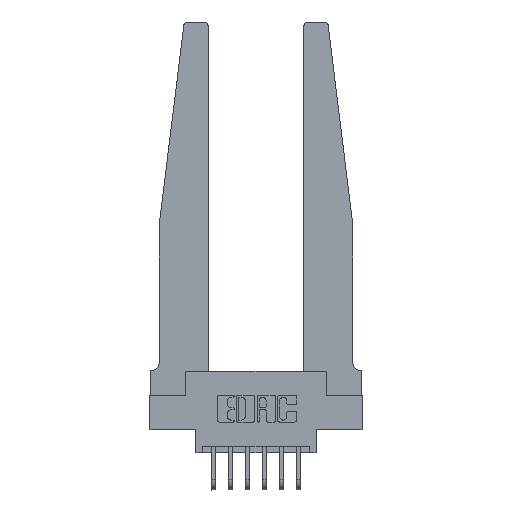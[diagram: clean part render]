
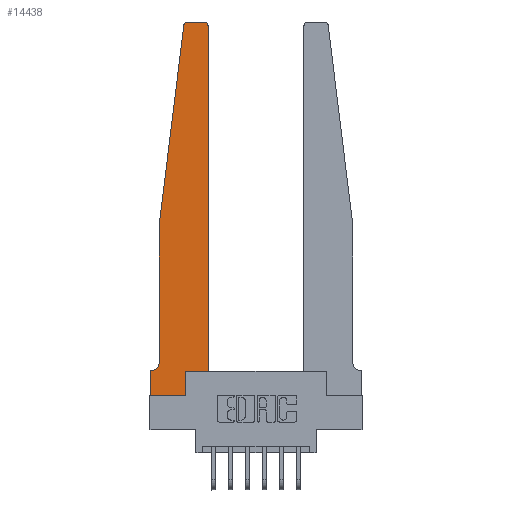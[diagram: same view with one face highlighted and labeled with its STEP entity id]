
A CAD part, top view. The second image highlights one B-rep face of the part: STEP entity #14438.
In plain terms, the highlighted planar face has unit normal (0, 0, 1).
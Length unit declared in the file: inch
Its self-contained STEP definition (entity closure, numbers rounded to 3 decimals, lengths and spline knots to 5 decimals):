
#33 = CARTESIAN_POINT ( 'NONE',  ( 0.2605, 0.18, 0.37 ) ) ;
#292 = CARTESIAN_POINT ( 'NONE',  ( 0.2605, 0.18, 0.37 ) ) ;
#530 = EDGE_CURVE ( 'NONE', #10565, #9992, #12898, .T. ) ;
#574 = ORIENTED_EDGE ( 'NONE', *, *, #530, .T. ) ;
#736 = CARTESIAN_POINT ( 'NONE',  ( 0.24675, 2.72367, 0.37 ) ) ;
#763 = VECTOR ( 'NONE', #12219, 39.37008 ) ;
#827 = VERTEX_POINT ( 'NONE', #8592 ) ;
#1291 = LINE ( 'NONE', #292, #8267 ) ;
#1582 = DIRECTION ( 'NONE',  ( 1., 0., 0. ) ) ;
#1612 = ORIENTED_EDGE ( 'NONE', *, *, #15298, .T. ) ;
#1615 = VERTEX_POINT ( 'NONE', #8436 ) ;
#1773 = EDGE_CURVE ( 'NONE', #827, #10565, #1291, .T. ) ;
#1791 = DIRECTION ( 'NONE',  ( 1., 0., 0. ) ) ;
#1896 = CIRCLE ( 'NONE', #10002, 0.05 ) ;
#2230 = LINE ( 'NONE', #6598, #2796 ) ;
#2315 = CARTESIAN_POINT ( 'NONE',  ( 0.27653, 2.75, 0.37 ) ) ;
#2355 = ORIENTED_EDGE ( 'NONE', *, *, #10225, .T. ) ;
#2376 = DIRECTION ( 'NONE',  ( 1., 0., 0. ) ) ;
#2778 = CARTESIAN_POINT ( 'NONE',  ( 0.425, 0.18, 0.37 ) ) ;
#2796 = VECTOR ( 'NONE', #7716, 39.37008 ) ;
#3054 = DIRECTION ( 'NONE',  ( -1., 0., 0. ) ) ;
#3140 = DIRECTION ( 'NONE',  ( 1., 0., 0. ) ) ;
#3184 = VERTEX_POINT ( 'NONE', #10871 ) ;
#3187 = DIRECTION ( 'NONE',  ( 0., -1., 0. ) ) ;
#3250 = CARTESIAN_POINT ( 'NONE',  ( 0., 0., 0.37 ) ) ;
#3554 = ORIENTED_EDGE ( 'NONE', *, *, #5472, .T. ) ;
#3602 = CARTESIAN_POINT ( 'NONE',  ( 0.27653, 2.72, 0.37 ) ) ;
#3672 = ORIENTED_EDGE ( 'NONE', *, *, #7025, .T. ) ;
#4065 = CARTESIAN_POINT ( 'NONE',  ( 0., 0., 0.37 ) ) ;
#4136 = FACE_OUTER_BOUND ( 'NONE', #4164, .T. ) ;
#4147 = CARTESIAN_POINT ( 'NONE',  ( 0.065, 1.25, 0.37 ) ) ;
#4158 = LINE ( 'NONE', #13344, #8698 ) ;
#4164 = EDGE_LOOP ( 'NONE', ( #13473, #2355, #3672, #8071, #6270, #7700, #9556, #3554, #5638, #574, #1612, #5847 ) ) ;
#4544 = AXIS2_PLACEMENT_3D ( 'NONE', #3602, #11991, #1582 ) ;
#4931 = VECTOR ( 'NONE', #11007, 39.37008 ) ;
#5241 = LINE ( 'NONE', #7638, #9429 ) ;
#5472 = EDGE_CURVE ( 'NONE', #8073, #827, #13823, .T. ) ;
#5638 = ORIENTED_EDGE ( 'NONE', *, *, #1773, .T. ) ;
#5847 = ORIENTED_EDGE ( 'NONE', *, *, #10850, .T. ) ;
#6134 = DIRECTION ( 'NONE',  ( 0., 1., 0. ) ) ;
#6270 = ORIENTED_EDGE ( 'NONE', *, *, #9929, .T. ) ;
#6478 = LINE ( 'NONE', #7479, #4931 ) ;
#6598 = CARTESIAN_POINT ( 'NONE',  ( 0.25, 2.75, 0.37 ) ) ;
#6753 = CARTESIAN_POINT ( 'NONE',  ( 0.395, 2.75, 0.37 ) ) ;
#6863 = PLANE ( 'NONE',  #7045 ) ;
#6876 = AXIS2_PLACEMENT_3D ( 'NONE', #14218, #14267, #2376 ) ;
#6998 = DIRECTION ( 'NONE',  ( 0., 0., -1. ) ) ;
#7025 = EDGE_CURVE ( 'NONE', #13683, #13902, #6478, .T. ) ;
#7045 = AXIS2_PLACEMENT_3D ( 'NONE', #9255, #7933, #3140 ) ;
#7364 = EDGE_CURVE ( 'NONE', #14016, #8073, #13776, .T. ) ;
#7479 = CARTESIAN_POINT ( 'NONE',  ( 0.065, 1.25, 0.37 ) ) ;
#7638 = CARTESIAN_POINT ( 'NONE',  ( 0.065, 1.25, 0.37 ) ) ;
#7700 = ORIENTED_EDGE ( 'NONE', *, *, #10220, .T. ) ;
#7716 = DIRECTION ( 'NONE',  ( -1., 0., 0. ) ) ;
#7933 = DIRECTION ( 'NONE',  ( 0., 0., 1. ) ) ;
#8071 = ORIENTED_EDGE ( 'NONE', *, *, #10265, .T. ) ;
#8073 = VERTEX_POINT ( 'NONE', #15427 ) ;
#8267 = VECTOR ( 'NONE', #6134, 39.37008 ) ;
#8436 = CARTESIAN_POINT ( 'NONE',  ( 0.425, 2.72, 0.37 ) ) ;
#8551 = CARTESIAN_POINT ( 'NONE',  ( 0.425, 0.18, 0.37 ) ) ;
#8592 = CARTESIAN_POINT ( 'NONE',  ( 0.2605, 0., 0.37 ) ) ;
#8613 = DIRECTION ( 'NONE',  ( 0., 1., 0. ) ) ;
#8698 = VECTOR ( 'NONE', #3054, 39.37008 ) ;
#9186 = EDGE_CURVE ( 'NONE', #10079, #9987, #2230, .T. ) ;
#9237 = CIRCLE ( 'NONE', #4544, 0.03 ) ;
#9255 = CARTESIAN_POINT ( 'NONE',  ( 0., 0.1875, 0.37 ) ) ;
#9429 = VECTOR ( 'NONE', #14999, 39.37008 ) ;
#9556 = ORIENTED_EDGE ( 'NONE', *, *, #7364, .T. ) ;
#9929 = EDGE_CURVE ( 'NONE', #3184, #10989, #1896, .T. ) ;
#9987 = VERTEX_POINT ( 'NONE', #2315 ) ;
#9992 = VERTEX_POINT ( 'NONE', #2778 ) ;
#10002 = AXIS2_PLACEMENT_3D ( 'NONE', #10705, #6998, #10599 ) ;
#10079 = VERTEX_POINT ( 'NONE', #6753 ) ;
#10220 = EDGE_CURVE ( 'NONE', #10989, #14016, #4158, .T. ) ;
#10225 = EDGE_CURVE ( 'NONE', #9987, #13683, #9237, .T. ) ;
#10265 = EDGE_CURVE ( 'NONE', #13902, #3184, #5241, .T. ) ;
#10428 = CARTESIAN_POINT ( 'NONE',  ( 0., 0.1875, 0.37 ) ) ;
#10565 = VERTEX_POINT ( 'NONE', #33 ) ;
#10599 = DIRECTION ( 'NONE',  ( -1., 0., 0. ) ) ;
#10705 = CARTESIAN_POINT ( 'NONE',  ( 0.015, 0.2375, 0.37 ) ) ;
#10850 = EDGE_CURVE ( 'NONE', #1615, #10079, #15074, .T. ) ;
#10871 = CARTESIAN_POINT ( 'NONE',  ( 0.065, 0.2375, 0.37 ) ) ;
#10989 = VERTEX_POINT ( 'NONE', #14539 ) ;
#11007 = DIRECTION ( 'NONE',  ( -0.122, -0.992, 0. ) ) ;
#11034 = CARTESIAN_POINT ( 'NONE',  ( 0.425, 0.18, 0.37 ) ) ;
#11481 = VECTOR ( 'NONE', #8613, 39.37008 ) ;
#11991 = DIRECTION ( 'NONE',  ( 0., 0., 1. ) ) ;
#12219 = DIRECTION ( 'NONE',  ( 1., 0., 0. ) ) ;
#12492 = VECTOR ( 'NONE', #3187, 39.37008 ) ;
#12898 = LINE ( 'NONE', #11034, #763 ) ;
#13344 = CARTESIAN_POINT ( 'NONE',  ( 0.065, 0.1875, 0.37 ) ) ;
#13473 = ORIENTED_EDGE ( 'NONE', *, *, #9186, .T. ) ;
#13625 = VECTOR ( 'NONE', #1791, 39.37008 ) ;
#13683 = VERTEX_POINT ( 'NONE', #736 ) ;
#13776 = LINE ( 'NONE', #3250, #12492 ) ;
#13823 = LINE ( 'NONE', #4065, #13625 ) ;
#13902 = VERTEX_POINT ( 'NONE', #4147 ) ;
#14016 = VERTEX_POINT ( 'NONE', #10428 ) ;
#14218 = CARTESIAN_POINT ( 'NONE',  ( 0.395, 2.72, 0.37 ) ) ;
#14267 = DIRECTION ( 'NONE',  ( 0., 0., 1. ) ) ;
#14438 = ADVANCED_FACE ( 'NONE', ( #4136 ), #6863, .T. ) ;
#14539 = CARTESIAN_POINT ( 'NONE',  ( 0.015, 0.1875, 0.37 ) ) ;
#14999 = DIRECTION ( 'NONE',  ( 0., -1., 0. ) ) ;
#15007 = LINE ( 'NONE', #8551, #11481 ) ;
#15074 = CIRCLE ( 'NONE', #6876, 0.03 ) ;
#15298 = EDGE_CURVE ( 'NONE', #9992, #1615, #15007, .T. ) ;
#15427 = CARTESIAN_POINT ( 'NONE',  ( 0., 0., 0.37 ) ) ;
